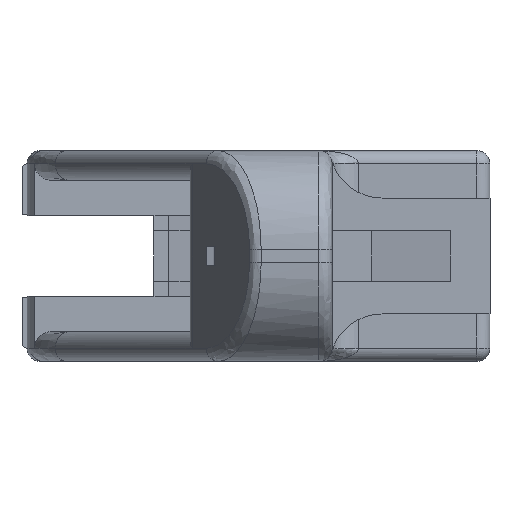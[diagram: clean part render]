
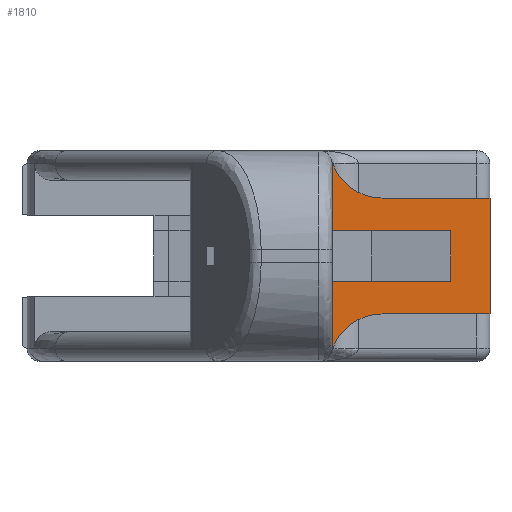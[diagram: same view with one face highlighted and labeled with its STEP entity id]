
A CAD part, left-side view. The second image highlights one B-rep face of the part: STEP entity #1810.
In plain terms, the highlighted planar face has unit normal (-1, 0, 0).
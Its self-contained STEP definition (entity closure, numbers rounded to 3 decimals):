
#167 = EDGE_LOOP ( 'NONE', ( #4840, #4847, #4865, #4832, #4834, #4854, #4859, #4845, #4838, #4846, #4858, #4855 ) ) ;
#1061 = CARTESIAN_POINT ( 'NONE',  ( -92.837, -22.86, 25.146 ) ) ;
#1067 = CARTESIAN_POINT ( 'NONE',  ( -92.837, -9.652, 31.496 ) ) ;
#1073 = CARTESIAN_POINT ( 'NONE',  ( -92.837, -30.48, 9.144 ) ) ;
#1075 = CARTESIAN_POINT ( 'NONE',  ( -92.837, -30.48, 31.496 ) ) ;
#1076 = CARTESIAN_POINT ( 'NONE',  ( -92.837, 0., 2.54 ) ) ;
#1080 = CARTESIAN_POINT ( 'NONE',  ( -92.837, 0., 38.1 ) ) ;
#1081 = CARTESIAN_POINT ( 'NONE',  ( -92.837, -9.652, 9.144 ) ) ;
#1099 = CARTESIAN_POINT ( 'NONE',  ( -92.837, 0., 15.494 ) ) ;
#1100 = CARTESIAN_POINT ( 'NONE',  ( -92.837, 0., 25.146 ) ) ;
#1108 = CARTESIAN_POINT ( 'NONE',  ( -92.837, 0.102, 1.829 ) ) ;
#1111 = CARTESIAN_POINT ( 'NONE',  ( -92.837, 0.102, 38.811 ) ) ;
#1113 = CARTESIAN_POINT ( 'NONE',  ( -92.837, -22.86, 15.494 ) ) ;
#1654 = EDGE_CURVE ( 'NONE', #5143, #5152, #2666, .T. ) ;
#1658 = EDGE_CURVE ( 'NONE', #5133, #5149, #2665, .T. ) ;
#1660 = EDGE_CURVE ( 'NONE', #5143, #5134, #2652, .T. ) ;
#1661 = EDGE_CURVE ( 'NONE', #5124, #5167, #2040, .T. ) ;
#1666 = EDGE_CURVE ( 'NONE', #5126, #5127, #2701, .T. ) ;
#1672 = EDGE_CURVE ( 'NONE', #5120, #5127, #2738, .T. ) ;
#1674 = EDGE_CURVE ( 'NONE', #5133, #5152, #2754, .T. ) ;
#1676 = EDGE_CURVE ( 'NONE', #5135, #5167, #2043, .T. ) ;
#1677 = EDGE_CURVE ( 'NONE', #5135, #5149, #2774, .T. ) ;
#1678 = EDGE_CURVE ( 'NONE', #5164, #5134, #2054, .T. ) ;
#1681 = EDGE_CURVE ( 'NONE', #5120, #5164, #2039, .T. ) ;
#1700 = EDGE_CURVE ( 'NONE', #5124, #5126, #2865, .T. ) ;
#1810 = ADVANCED_FACE ( 'NONE', ( #6080 ), #3547, .F. ) ;
#2039 = CIRCLE ( 'NONE', #5909, 10.16 ) ;
#2040 = CIRCLE ( 'NONE', #5885, 10.16 ) ;
#2043 = CIRCLE ( 'NONE', #5895, 2.54 ) ;
#2054 = CIRCLE ( 'NONE', #5894, 2.54 ) ;
#2622 = CARTESIAN_POINT ( 'NONE',  ( -92.837, -9.652, 41.656 ) ) ;
#2646 = CARTESIAN_POINT ( 'NONE',  ( -92.837, -22.86, 25.146 ) ) ;
#2650 = DIRECTION ( 'NONE',  ( 0., -1., 0. ) ) ;
#2652 = LINE ( 'NONE', #2654, #5902 ) ;
#2654 = CARTESIAN_POINT ( 'NONE',  ( -92.837, 0., 40.64 ) ) ;
#2656 = DIRECTION ( 'NONE',  ( 0., 0., -1. ) ) ;
#2657 = DIRECTION ( 'NONE',  ( 1., 0., 0. ) ) ;
#2659 = DIRECTION ( 'NONE',  ( 0., 1., 0. ) ) ;
#2660 = CARTESIAN_POINT ( 'NONE',  ( -92.837, -22.86, 15.494 ) ) ;
#2665 = LINE ( 'NONE', #2646, #5900 ) ;
#2666 = LINE ( 'NONE', #2660, #5888 ) ;
#2674 = DIRECTION ( 'NONE',  ( 0., -1., 0. ) ) ;
#2690 = DIRECTION ( 'NONE',  ( 0., 0., -1. ) ) ;
#2697 = CARTESIAN_POINT ( 'NONE',  ( -92.837, -30.48, 9.144 ) ) ;
#2701 = LINE ( 'NONE', #2697, #5890 ) ;
#2734 = CARTESIAN_POINT ( 'NONE',  ( -92.837, -22.86, 9.144 ) ) ;
#2735 = DIRECTION ( 'NONE',  ( 0., -1., 0. ) ) ;
#2738 = LINE ( 'NONE', #2734, #5916 ) ;
#2753 = CARTESIAN_POINT ( 'NONE',  ( -92.837, -22.86, 9.144 ) ) ;
#2754 = LINE ( 'NONE', #2753, #5911 ) ;
#2757 = DIRECTION ( 'NONE',  ( 0., 0., -1. ) ) ;
#2761 = CARTESIAN_POINT ( 'NONE',  ( -92.837, 2.54, 38.1 ) ) ;
#2762 = DIRECTION ( 'NONE',  ( -1., 0., 0. ) ) ;
#2763 = DIRECTION ( 'NONE',  ( 0., -1., 0. ) ) ;
#2764 = CARTESIAN_POINT ( 'NONE',  ( -92.837, 2.54, 2.54 ) ) ;
#2769 = DIRECTION ( 'NONE',  ( -1., 0., 0. ) ) ;
#2770 = DIRECTION ( 'NONE',  ( 0., 0., -1. ) ) ;
#2771 = DIRECTION ( 'NONE',  ( 0., 1., 0. ) ) ;
#2773 = CARTESIAN_POINT ( 'NONE',  ( -92.837, 0., 40.64 ) ) ;
#2774 = LINE ( 'NONE', #2773, #5910 ) ;
#2775 = DIRECTION ( 'NONE',  ( -1., 0., 0. ) ) ;
#2777 = CARTESIAN_POINT ( 'NONE',  ( -92.837, -9.652, -1.016 ) ) ;
#2778 = DIRECTION ( 'NONE',  ( 0., 1., 0. ) ) ;
#2865 = LINE ( 'NONE', #2870, #5931 ) ;
#2870 = CARTESIAN_POINT ( 'NONE',  ( -92.837, -22.86, 31.496 ) ) ;
#2872 = DIRECTION ( 'NONE',  ( 0., -1., 0. ) ) ;
#2953 = CARTESIAN_POINT ( 'NONE',  ( -92.837, -22.86, 15.494 ) ) ;
#2956 = DIRECTION ( 'NONE',  ( 1., 0., 0. ) ) ;
#2961 = DIRECTION ( 'NONE',  ( 0., 1., 0. ) ) ;
#3547 = PLANE ( 'NONE',  #6111 ) ;
#4832 = ORIENTED_EDGE ( 'NONE', *, *, #1661, .T. ) ;
#4834 = ORIENTED_EDGE ( 'NONE', *, *, #1676, .F. ) ;
#4838 = ORIENTED_EDGE ( 'NONE', *, *, #1654, .F. ) ;
#4840 = ORIENTED_EDGE ( 'NONE', *, *, #1672, .T. ) ;
#4845 = ORIENTED_EDGE ( 'NONE', *, *, #1674, .T. ) ;
#4846 = ORIENTED_EDGE ( 'NONE', *, *, #1660, .T. ) ;
#4847 = ORIENTED_EDGE ( 'NONE', *, *, #1666, .F. ) ;
#4854 = ORIENTED_EDGE ( 'NONE', *, *, #1677, .T. ) ;
#4855 = ORIENTED_EDGE ( 'NONE', *, *, #1681, .F. ) ;
#4858 = ORIENTED_EDGE ( 'NONE', *, *, #1678, .F. ) ;
#4859 = ORIENTED_EDGE ( 'NONE', *, *, #1658, .F. ) ;
#4865 = ORIENTED_EDGE ( 'NONE', *, *, #1700, .F. ) ;
#5120 = VERTEX_POINT ( 'NONE', #1081 ) ;
#5124 = VERTEX_POINT ( 'NONE', #1067 ) ;
#5126 = VERTEX_POINT ( 'NONE', #1075 ) ;
#5127 = VERTEX_POINT ( 'NONE', #1073 ) ;
#5133 = VERTEX_POINT ( 'NONE', #1061 ) ;
#5134 = VERTEX_POINT ( 'NONE', #1076 ) ;
#5135 = VERTEX_POINT ( 'NONE', #1080 ) ;
#5143 = VERTEX_POINT ( 'NONE', #1099 ) ;
#5149 = VERTEX_POINT ( 'NONE', #1100 ) ;
#5152 = VERTEX_POINT ( 'NONE', #1113 ) ;
#5164 = VERTEX_POINT ( 'NONE', #1108 ) ;
#5167 = VERTEX_POINT ( 'NONE', #1111 ) ;
#5885 = AXIS2_PLACEMENT_3D ( 'NONE', #2622, #2657, #2674 ) ;
#5888 = VECTOR ( 'NONE', #2650, 1000. ) ;
#5890 = VECTOR ( 'NONE', #2690, 1000. ) ;
#5894 = AXIS2_PLACEMENT_3D ( 'NONE', #2764, #2769, #2771 ) ;
#5895 = AXIS2_PLACEMENT_3D ( 'NONE', #2761, #2762, #2763 ) ;
#5900 = VECTOR ( 'NONE', #2659, 1000. ) ;
#5902 = VECTOR ( 'NONE', #2656, 1000. ) ;
#5909 = AXIS2_PLACEMENT_3D ( 'NONE', #2777, #2775, #2778 ) ;
#5910 = VECTOR ( 'NONE', #2770, 1000. ) ;
#5911 = VECTOR ( 'NONE', #2757, 1000. ) ;
#5916 = VECTOR ( 'NONE', #2735, 1000. ) ;
#5931 = VECTOR ( 'NONE', #2872, 1000. ) ;
#6080 = FACE_OUTER_BOUND ( 'NONE', #167, .T. ) ;
#6111 = AXIS2_PLACEMENT_3D ( 'NONE', #2953, #2956, #2961 ) ;
